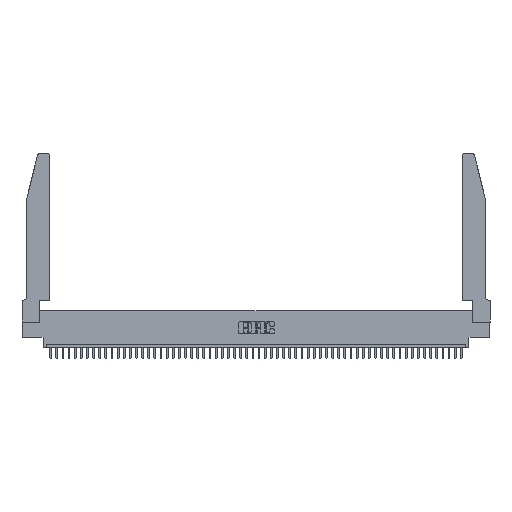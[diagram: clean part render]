
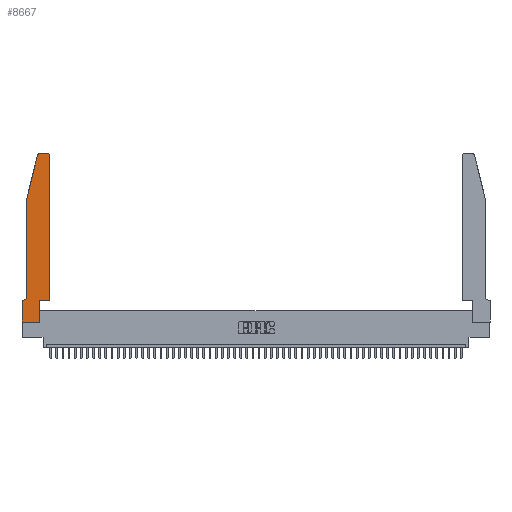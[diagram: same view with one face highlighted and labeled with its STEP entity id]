
A CAD part, top view. The second image highlights one B-rep face of the part: STEP entity #8667.
In plain terms, the highlighted planar face has unit normal (0, 0, 1).
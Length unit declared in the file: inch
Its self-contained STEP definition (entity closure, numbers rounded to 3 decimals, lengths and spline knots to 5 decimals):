
#158 = CARTESIAN_POINT ( 'NONE',  ( 0.0755, 0.35, 0.37 ) ) ;
#1846 = CIRCLE ( 'NONE', #45640, 0.03 ) ;
#2531 = VERTEX_POINT ( 'NONE', #44834 ) ;
#2642 = ORIENTED_EDGE ( 'NONE', *, *, #46340, .T. ) ;
#3201 = CARTESIAN_POINT ( 'NONE',  ( 0., 0., 0.37 ) ) ;
#3834 = LINE ( 'NONE', #42480, #17784 ) ;
#5044 = VERTEX_POINT ( 'NONE', #10389 ) ;
#5435 = CARTESIAN_POINT ( 'NONE',  ( 0.4505, 2.72, 0.37 ) ) ;
#6623 = VERTEX_POINT ( 'NONE', #43924 ) ;
#7164 = ORIENTED_EDGE ( 'NONE', *, *, #27575, .T. ) ;
#7616 = ORIENTED_EDGE ( 'NONE', *, *, #9788, .T. ) ;
#7944 = DIRECTION ( 'NONE',  ( 0., 1., 0. ) ) ;
#8667 = ADVANCED_FACE ( 'NONE', ( #15775 ), #19294, .T. ) ;
#9467 = AXIS2_PLACEMENT_3D ( 'NONE', #28754, #28930, #45669 ) ;
#9490 = CIRCLE ( 'NONE', #9467, 0.03 ) ;
#9788 = EDGE_CURVE ( 'NONE', #5044, #17919, #42938, .T. ) ;
#9939 = EDGE_LOOP ( 'NONE', ( #26002, #47682, #12283, #13507, #7616, #2642, #16559, #7164, #13959, #26114, #39024, #11872 ) ) ;
#10389 = CARTESIAN_POINT ( 'NONE',  ( 0.0755, 0.42, 0.37 ) ) ;
#10616 = DIRECTION ( 'NONE',  ( 0., -1., 0. ) ) ;
#10680 = CARTESIAN_POINT ( 'NONE',  ( 0.0055, 0.42, 0.37 ) ) ;
#10857 = LINE ( 'NONE', #27257, #50861 ) ;
#11872 = ORIENTED_EDGE ( 'NONE', *, *, #32943, .T. ) ;
#12283 = ORIENTED_EDGE ( 'NONE', *, *, #35731, .T. ) ;
#12867 = AXIS2_PLACEMENT_3D ( 'NONE', #38949, #51801, #43056 ) ;
#13096 = VECTOR ( 'NONE', #7944, 39.37008 ) ;
#13507 = ORIENTED_EDGE ( 'NONE', *, *, #27665, .T. ) ;
#13568 = VERTEX_POINT ( 'NONE', #23031 ) ;
#13605 = CARTESIAN_POINT ( 'NONE',  ( 0., 0., 0.37 ) ) ;
#13959 = ORIENTED_EDGE ( 'NONE', *, *, #20386, .T. ) ;
#15130 = DIRECTION ( 'NONE',  ( -1., 0., 0. ) ) ;
#15427 = CARTESIAN_POINT ( 'NONE',  ( 0.0755, 2., 0.37 ) ) ;
#15775 = FACE_OUTER_BOUND ( 'NONE', #9939, .T. ) ;
#16534 = EDGE_CURVE ( 'NONE', #6623, #44715, #30895, .T. ) ;
#16559 = ORIENTED_EDGE ( 'NONE', *, *, #20328, .T. ) ;
#16572 = LINE ( 'NONE', #15427, #21605 ) ;
#16607 = VERTEX_POINT ( 'NONE', #21697 ) ;
#17784 = VECTOR ( 'NONE', #46570, 39.37008 ) ;
#17919 = VERTEX_POINT ( 'NONE', #43737 ) ;
#19294 = PLANE ( 'NONE',  #12867 ) ;
#19531 = VECTOR ( 'NONE', #36356, 39.37008 ) ;
#20328 = EDGE_CURVE ( 'NONE', #40425, #22540, #29635, .T. ) ;
#20386 = EDGE_CURVE ( 'NONE', #2531, #35574, #45580, .T. ) ;
#21193 = CARTESIAN_POINT ( 'NONE',  ( 0., 0.35, 0.37 ) ) ;
#21404 = VECTOR ( 'NONE', #10616, 39.37008 ) ;
#21561 = CARTESIAN_POINT ( 'NONE',  ( 0.2865, 0.35, 0.37 ) ) ;
#21605 = VECTOR ( 'NONE', #40247, 39.37008 ) ;
#21697 = CARTESIAN_POINT ( 'NONE',  ( 0.25487, 2.72718, 0.37 ) ) ;
#22540 = VERTEX_POINT ( 'NONE', #49067 ) ;
#23031 = CARTESIAN_POINT ( 'NONE',  ( 0.284, 2.75, 0.37 ) ) ;
#23393 = DIRECTION ( 'NONE',  ( 1., 0., 0. ) ) ;
#23509 = LINE ( 'NONE', #13605, #52174 ) ;
#23787 = DIRECTION ( 'NONE',  ( 1., 0., 0. ) ) ;
#24299 = DIRECTION ( 'NONE',  ( -1., 0., 0. ) ) ;
#25575 = DIRECTION ( 'NONE',  ( 1., 0., 0. ) ) ;
#26002 = ORIENTED_EDGE ( 'NONE', *, *, #44949, .T. ) ;
#26114 = ORIENTED_EDGE ( 'NONE', *, *, #51242, .T. ) ;
#27257 = CARTESIAN_POINT ( 'NONE',  ( 0.4505, 0.35, 0.37 ) ) ;
#27575 = EDGE_CURVE ( 'NONE', #22540, #2531, #23509, .T. ) ;
#27601 = VERTEX_POINT ( 'NONE', #31354 ) ;
#27665 = EDGE_CURVE ( 'NONE', #51533, #5044, #3834, .T. ) ;
#27695 = CARTESIAN_POINT ( 'NONE',  ( 0.0755, 2., 0.37 ) ) ;
#28754 = CARTESIAN_POINT ( 'NONE',  ( 0.284, 2.72, 0.37 ) ) ;
#28930 = DIRECTION ( 'NONE',  ( 0., 0., 1. ) ) ;
#29635 = LINE ( 'NONE', #3201, #21404 ) ;
#30644 = CARTESIAN_POINT ( 'NONE',  ( 0.2865, 0.35, 0.37 ) ) ;
#30895 = LINE ( 'NONE', #48577, #13096 ) ;
#31354 = CARTESIAN_POINT ( 'NONE',  ( 0.4205, 2.75, 0.37 ) ) ;
#32299 = DIRECTION ( 'NONE',  ( 0., 0., 1. ) ) ;
#32943 = EDGE_CURVE ( 'NONE', #44715, #27601, #1846, .T. ) ;
#35396 = AXIS2_PLACEMENT_3D ( 'NONE', #10680, #39600, #15130 ) ;
#35574 = VERTEX_POINT ( 'NONE', #30644 ) ;
#35685 = CARTESIAN_POINT ( 'NONE',  ( 0.2605, 2.75, 0.37 ) ) ;
#35731 = EDGE_CURVE ( 'NONE', #16607, #51533, #16572, .T. ) ;
#36356 = DIRECTION ( 'NONE',  ( -1., 0., 0. ) ) ;
#36425 = VECTOR ( 'NONE', #24299, 39.37008 ) ;
#37793 = LINE ( 'NONE', #35685, #19531 ) ;
#38949 = CARTESIAN_POINT ( 'NONE',  ( 0., 0.35, 0.37 ) ) ;
#39024 = ORIENTED_EDGE ( 'NONE', *, *, #16534, .T. ) ;
#39600 = DIRECTION ( 'NONE',  ( 0., 0., -1. ) ) ;
#40247 = DIRECTION ( 'NONE',  ( -0.239, -0.971, 0. ) ) ;
#40425 = VERTEX_POINT ( 'NONE', #21193 ) ;
#42367 = EDGE_CURVE ( 'NONE', #13568, #16607, #9490, .T. ) ;
#42480 = CARTESIAN_POINT ( 'NONE',  ( 0.0755, 2., 0.37 ) ) ;
#42938 = CIRCLE ( 'NONE', #35396, 0.07 ) ;
#43056 = DIRECTION ( 'NONE',  ( 1., 0., 0. ) ) ;
#43723 = CARTESIAN_POINT ( 'NONE',  ( 0.4205, 2.72, 0.37 ) ) ;
#43737 = CARTESIAN_POINT ( 'NONE',  ( 0.0055, 0.35, 0.37 ) ) ;
#43924 = CARTESIAN_POINT ( 'NONE',  ( 0.4505, 0.35, 0.37 ) ) ;
#44715 = VERTEX_POINT ( 'NONE', #5435 ) ;
#44834 = CARTESIAN_POINT ( 'NONE',  ( 0.2865, 0., 0.37 ) ) ;
#44949 = EDGE_CURVE ( 'NONE', #27601, #13568, #37793, .T. ) ;
#45580 = LINE ( 'NONE', #21561, #49429 ) ;
#45640 = AXIS2_PLACEMENT_3D ( 'NONE', #43723, #32299, #23787 ) ;
#45669 = DIRECTION ( 'NONE',  ( 1., 0., 0. ) ) ;
#46340 = EDGE_CURVE ( 'NONE', #17919, #40425, #47291, .T. ) ;
#46570 = DIRECTION ( 'NONE',  ( 0., -1., 0. ) ) ;
#47291 = LINE ( 'NONE', #158, #36425 ) ;
#47682 = ORIENTED_EDGE ( 'NONE', *, *, #42367, .T. ) ;
#48577 = CARTESIAN_POINT ( 'NONE',  ( 0.4505, 0.35, 0.37 ) ) ;
#49067 = CARTESIAN_POINT ( 'NONE',  ( 0., 0., 0.37 ) ) ;
#49429 = VECTOR ( 'NONE', #51853, 39.37008 ) ;
#50861 = VECTOR ( 'NONE', #23393, 39.37008 ) ;
#51242 = EDGE_CURVE ( 'NONE', #35574, #6623, #10857, .T. ) ;
#51533 = VERTEX_POINT ( 'NONE', #27695 ) ;
#51801 = DIRECTION ( 'NONE',  ( 0., 0., 1. ) ) ;
#51853 = DIRECTION ( 'NONE',  ( 0., 1., 0. ) ) ;
#52174 = VECTOR ( 'NONE', #25575, 39.37008 ) ;
